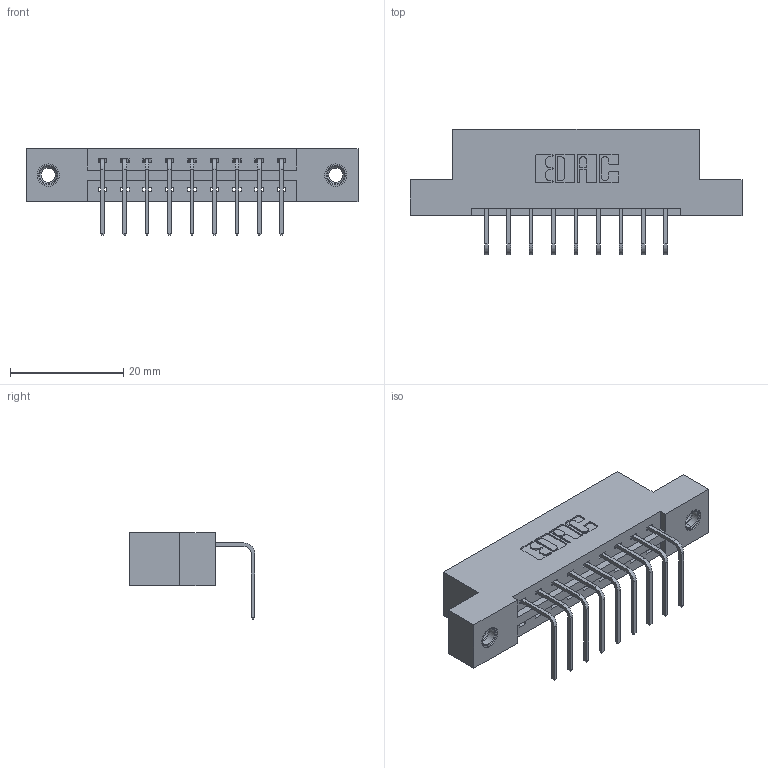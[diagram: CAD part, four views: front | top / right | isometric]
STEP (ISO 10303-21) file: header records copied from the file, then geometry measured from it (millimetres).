
FILE_DESCRIPTION (( 'STEP AP203' ), '1' );
FILE_NAME ('337-009-558-107.STEP', '2019-10-07T11:19:23', ( '' ), ( '' ), 'SwSTEP 2.0', 'SolidWorks 2016', '' );
FILE_SCHEMA (( 'CONFIG_CONTROL_DESIGN' ));
Length unit declared in the file: inch
Products named in the file (4): 337 Part_Flush Mounting Lugs - 0.156 Dia-TI; 337-009-558-107; 345-250-001_345-250-005-103; 345-292-001_558 Tail - 2
Assembly tree (12 placements, depth 2):
  337-009-558-107
    337 Part_Flush Mounting Lugs - 0.156 Dia-TI
    345-292-001_558 Tail - 2  x9
    345-250-001_345-250-005-103  x2
Bounding box: 58.67 x 22.17 x 15.37 mm (x, y, z)
Volume: 5701.7 mm3; surface area: 5934 mm2
Topology: 12 solids, 12 shells, 750 faces, 2193 edges, 1442 vertices
Faces by surface type: plane 534, cylinder 200, cone 12, torus 4
Entity records: 12228 total; most frequent: CARTESIAN_POINT 2108, ORIENTED_EDGE 2046, DIRECTION 1875, EDGE_CURVE 1023, VECTOR 875, LINE 875, VERTEX_POINT 676, AXIS2_PLACEMENT_3D 500
